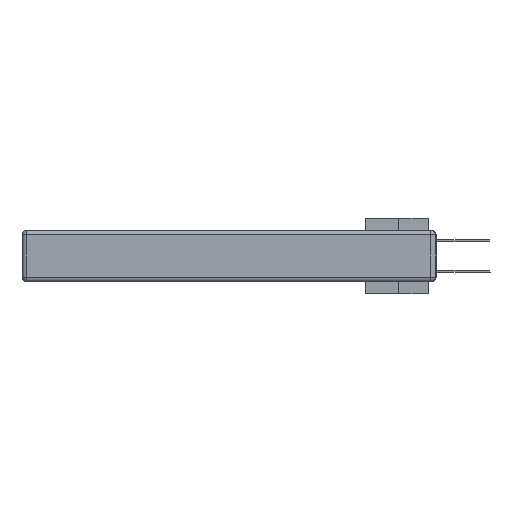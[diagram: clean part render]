
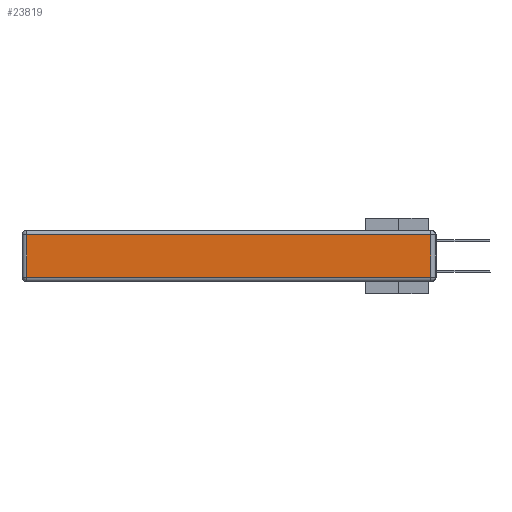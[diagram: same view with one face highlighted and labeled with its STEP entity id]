
A CAD part, left-side view. The second image highlights one B-rep face of the part: STEP entity #23819.
In plain terms, the highlighted planar face has unit normal (-1, 0, 0).
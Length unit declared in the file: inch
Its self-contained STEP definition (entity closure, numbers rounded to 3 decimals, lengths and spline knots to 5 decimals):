
#1109 = AXIS2_PLACEMENT_3D ( 'NONE', #3581, #21158, #6110 ) ;
#2211 = VERTEX_POINT ( 'NONE', #20904 ) ;
#2432 = ORIENTED_EDGE ( 'NONE', *, *, #27217, .T. ) ;
#3323 = LINE ( 'NONE', #23942, #13223 ) ;
#3581 = CARTESIAN_POINT ( 'NONE',  ( 0., 0., -0.343 ) ) ;
#4192 = VERTEX_POINT ( 'NONE', #8907 ) ;
#6110 = DIRECTION ( 'NONE',  ( 0., 0., 1. ) ) ;
#6840 = CARTESIAN_POINT ( 'NONE',  ( 0., 2.75, -0.03 ) ) ;
#7018 = ORIENTED_EDGE ( 'NONE', *, *, #27132, .T. ) ;
#7391 = VECTOR ( 'NONE', #16763, 39.37008 ) ;
#8907 = CARTESIAN_POINT ( 'NONE',  ( 0., 0.03, -0.313 ) ) ;
#9892 = ORIENTED_EDGE ( 'NONE', *, *, #29152, .T. ) ;
#10336 = VERTEX_POINT ( 'NONE', #13992 ) ;
#10562 = FACE_OUTER_BOUND ( 'NONE', #30752, .T. ) ;
#10631 = VECTOR ( 'NONE', #24460, 39.37008 ) ;
#11244 = CARTESIAN_POINT ( 'NONE',  ( 0., 2.72, -0.343 ) ) ;
#11370 = VECTOR ( 'NONE', #31441, 39.37008 ) ;
#12124 = LINE ( 'NONE', #6840, #7391 ) ;
#12399 = ORIENTED_EDGE ( 'NONE', *, *, #25952, .T. ) ;
#13223 = VECTOR ( 'NONE', #28816, 39.37008 ) ;
#13992 = CARTESIAN_POINT ( 'NONE',  ( 0., 2.72, -0.313 ) ) ;
#16763 = DIRECTION ( 'NONE',  ( 0., 1., 0. ) ) ;
#18461 = VERTEX_POINT ( 'NONE', #20083 ) ;
#20083 = CARTESIAN_POINT ( 'NONE',  ( 0., 0.03, -0.03 ) ) ;
#20904 = CARTESIAN_POINT ( 'NONE',  ( 0., 2.72, -0.03 ) ) ;
#21158 = DIRECTION ( 'NONE',  ( -1., 0., 0. ) ) ;
#22804 = LINE ( 'NONE', #24871, #10631 ) ;
#23819 = ADVANCED_FACE ( 'NONE', ( #10562 ), #26059, .T. ) ;
#23942 = CARTESIAN_POINT ( 'NONE',  ( 0., 0., -0.313 ) ) ;
#24460 = DIRECTION ( 'NONE',  ( 0., 0., 1. ) ) ;
#24871 = CARTESIAN_POINT ( 'NONE',  ( 0., 0.03, -0.343 ) ) ;
#25952 = EDGE_CURVE ( 'NONE', #4192, #18461, #22804, .T. ) ;
#26059 = PLANE ( 'NONE',  #1109 ) ;
#27132 = EDGE_CURVE ( 'NONE', #2211, #10336, #30082, .T. ) ;
#27217 = EDGE_CURVE ( 'NONE', #18461, #2211, #12124, .T. ) ;
#28816 = DIRECTION ( 'NONE',  ( 0., -1., 0. ) ) ;
#29152 = EDGE_CURVE ( 'NONE', #10336, #4192, #3323, .T. ) ;
#30082 = LINE ( 'NONE', #11244, #11370 ) ;
#30752 = EDGE_LOOP ( 'NONE', ( #9892, #12399, #2432, #7018 ) ) ;
#31441 = DIRECTION ( 'NONE',  ( 0., 0., -1. ) ) ;
